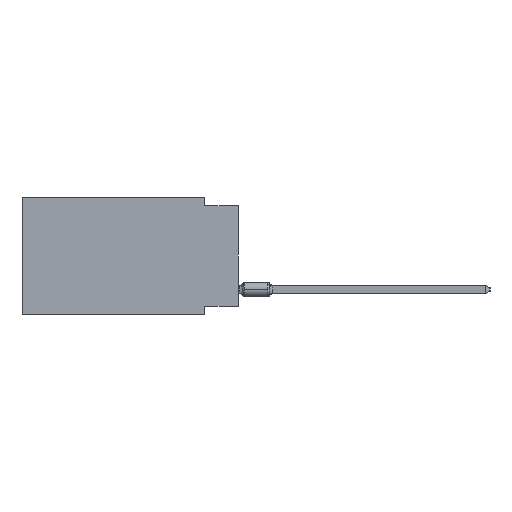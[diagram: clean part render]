
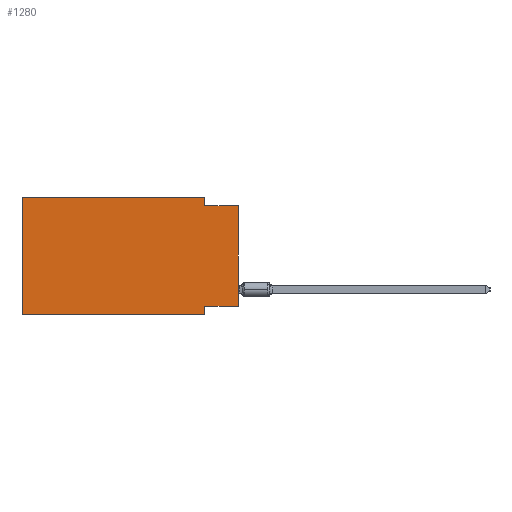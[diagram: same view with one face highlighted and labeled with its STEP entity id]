
A CAD part, left-side view. The second image highlights one B-rep face of the part: STEP entity #1280.
In plain terms, the highlighted planar face has unit normal (-1, 0, 0).
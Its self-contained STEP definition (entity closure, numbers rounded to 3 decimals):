
#73 = EDGE_CURVE ( 'NONE', #18673, #27883, #10777, .T. ) ;
#106 = DIRECTION ( 'NONE',  ( 0., 0., -1. ) ) ;
#231 = LINE ( 'NONE', #834, #19226 ) ;
#834 = CARTESIAN_POINT ( 'NONE',  ( 0., 0., -0.635 ) ) ;
#1065 = EDGE_CURVE ( 'NONE', #18673, #28784, #1308, .T. ) ;
#1280 = ADVANCED_FACE ( 'NONE', ( #29227 ), #14638, .F. ) ;
#1308 = LINE ( 'NONE', #5801, #21588 ) ;
#1519 = VERTEX_POINT ( 'NONE', #18447 ) ;
#1835 = VECTOR ( 'NONE', #17837, 1000. ) ;
#1985 = ORIENTED_EDGE ( 'NONE', *, *, #1065, .T. ) ;
#4218 = CARTESIAN_POINT ( 'NONE',  ( 0., 16.383, 0. ) ) ;
#4816 = DIRECTION ( 'NONE',  ( 0., 0., 1. ) ) ;
#5030 = CARTESIAN_POINT ( 'NONE',  ( 0., 16.383, 0. ) ) ;
#5358 = EDGE_CURVE ( 'NONE', #20608, #11242, #16811, .T. ) ;
#5608 = CARTESIAN_POINT ( 'NONE',  ( 0., 16.383, -8.89 ) ) ;
#5801 = CARTESIAN_POINT ( 'NONE',  ( 0., 0., 0. ) ) ;
#5857 = ORIENTED_EDGE ( 'NONE', *, *, #12877, .F. ) ;
#7814 = VECTOR ( 'NONE', #4816, 1000. ) ;
#7927 = LINE ( 'NONE', #5608, #24371 ) ;
#8508 = VECTOR ( 'NONE', #11180, 1000. ) ;
#8620 = LINE ( 'NONE', #15686, #24781 ) ;
#9065 = EDGE_CURVE ( 'NONE', #9703, #28784, #231, .T. ) ;
#9592 = EDGE_LOOP ( 'NONE', ( #1985, #18184, #14051, #19154, #20709, #30436, #5857, #28950 ) ) ;
#9703 = VERTEX_POINT ( 'NONE', #14334 ) ;
#9881 = CARTESIAN_POINT ( 'NONE',  ( 0., 16.383, 0. ) ) ;
#10569 = LINE ( 'NONE', #4218, #8508 ) ;
#10777 = LINE ( 'NONE', #20159, #1835 ) ;
#10950 = VERTEX_POINT ( 'NONE', #21997 ) ;
#11180 = DIRECTION ( 'NONE',  ( 0., -1., 0. ) ) ;
#11242 = VERTEX_POINT ( 'NONE', #5030 ) ;
#11437 = EDGE_CURVE ( 'NONE', #11242, #10950, #10569, .T. ) ;
#12215 = CARTESIAN_POINT ( 'NONE',  ( 0., 16.383, 0. ) ) ;
#12775 = EDGE_CURVE ( 'NONE', #10950, #9703, #8620, .T. ) ;
#12877 = EDGE_CURVE ( 'NONE', #27883, #1519, #28008, .T. ) ;
#14051 = ORIENTED_EDGE ( 'NONE', *, *, #12775, .F. ) ;
#14334 = CARTESIAN_POINT ( 'NONE',  ( 0., 2.54, -0.635 ) ) ;
#14638 = PLANE ( 'NONE',  #30434 ) ;
#14931 = DIRECTION ( 'NONE',  ( 0., 0., -1. ) ) ;
#15187 = DIRECTION ( 'NONE',  ( 0., 0., 1. ) ) ;
#15434 = VECTOR ( 'NONE', #106, 1000. ) ;
#15686 = CARTESIAN_POINT ( 'NONE',  ( 0., 2.54, 0. ) ) ;
#16811 = LINE ( 'NONE', #12215, #7814 ) ;
#17837 = DIRECTION ( 'NONE',  ( 0., 1., 0. ) ) ;
#18184 = ORIENTED_EDGE ( 'NONE', *, *, #9065, .F. ) ;
#18447 = CARTESIAN_POINT ( 'NONE',  ( 0., 2.54, -8.89 ) ) ;
#18673 = VERTEX_POINT ( 'NONE', #23023 ) ;
#19154 = ORIENTED_EDGE ( 'NONE', *, *, #11437, .F. ) ;
#19226 = VECTOR ( 'NONE', #23672, 1000. ) ;
#20159 = CARTESIAN_POINT ( 'NONE',  ( 0., 0., -8.255 ) ) ;
#20160 = CARTESIAN_POINT ( 'NONE',  ( 0., 2.54, -8.255 ) ) ;
#20608 = VERTEX_POINT ( 'NONE', #29560 ) ;
#20709 = ORIENTED_EDGE ( 'NONE', *, *, #5358, .F. ) ;
#20775 = CARTESIAN_POINT ( 'NONE',  ( 0., 2.54, -8.89 ) ) ;
#21588 = VECTOR ( 'NONE', #15187, 1000. ) ;
#21997 = CARTESIAN_POINT ( 'NONE',  ( 0., 2.54, 0. ) ) ;
#23023 = CARTESIAN_POINT ( 'NONE',  ( 0., 0., -8.255 ) ) ;
#23046 = EDGE_CURVE ( 'NONE', #20608, #1519, #7927, .T. ) ;
#23672 = DIRECTION ( 'NONE',  ( 0., -1., 0. ) ) ;
#24371 = VECTOR ( 'NONE', #24837, 1000. ) ;
#24781 = VECTOR ( 'NONE', #29394, 1000. ) ;
#24837 = DIRECTION ( 'NONE',  ( 0., -1., 0. ) ) ;
#26626 = DIRECTION ( 'NONE',  ( 1., 0., 0. ) ) ;
#27611 = CARTESIAN_POINT ( 'NONE',  ( 0., 0., -0.635 ) ) ;
#27883 = VERTEX_POINT ( 'NONE', #20160 ) ;
#28008 = LINE ( 'NONE', #20775, #15434 ) ;
#28784 = VERTEX_POINT ( 'NONE', #27611 ) ;
#28950 = ORIENTED_EDGE ( 'NONE', *, *, #73, .F. ) ;
#29227 = FACE_OUTER_BOUND ( 'NONE', #9592, .T. ) ;
#29394 = DIRECTION ( 'NONE',  ( 0., 0., -1. ) ) ;
#29560 = CARTESIAN_POINT ( 'NONE',  ( 0., 16.383, -8.89 ) ) ;
#30434 = AXIS2_PLACEMENT_3D ( 'NONE', #9881, #26626, #14931 ) ;
#30436 = ORIENTED_EDGE ( 'NONE', *, *, #23046, .T. ) ;
